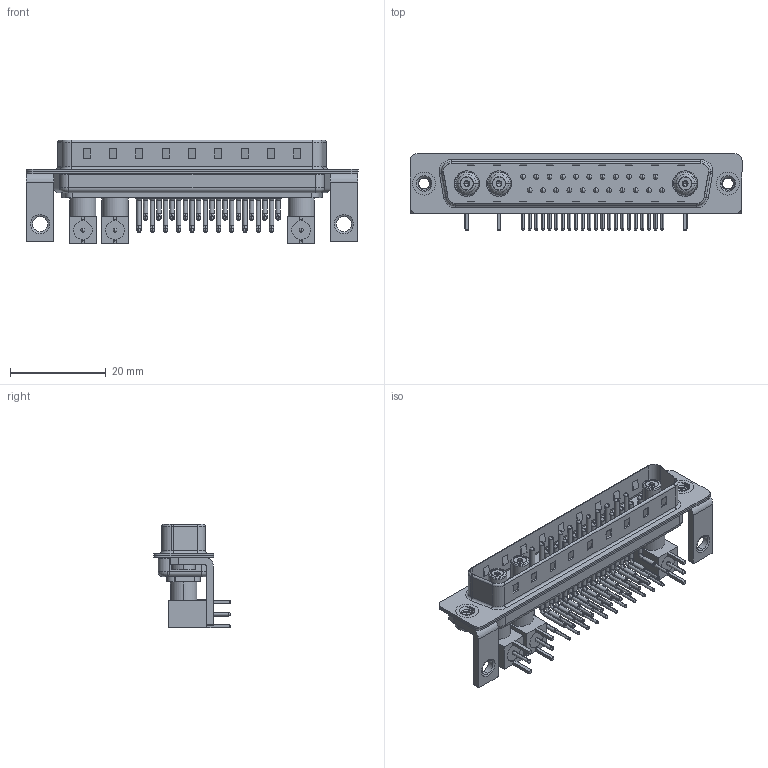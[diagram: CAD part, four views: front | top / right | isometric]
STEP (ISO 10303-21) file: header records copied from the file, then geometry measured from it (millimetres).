
FILE_DESCRIPTION (( 'STEP AP203' ), '1' );
FILE_NAME ('629-25W3640-7NC.STEP', '2022-05-16T09:23:09', ( '' ), ( '' ), 'SwSTEP 2.0', 'SolidWorks 2020', '' );
FILE_SCHEMA (( 'CONFIG_CONTROL_DESIGN' ));
Length unit declared in the file: millimetre
Products named in the file (18): 629Combo Threaded Rivet_2; Insulator RA Pin; 629Combo Shell Front_37 Contacts; Co-Ax Jack Assy_RA; 629Combo Stabilizer Bracket; 629-25W3640-7NC; 629Combo Housing_25W3; Co-Ax Jack_RA PC Tail; 629Combo Shell Rear_37 Contacts; Socket_RA; 629Combo Contact Row 2; Insulator Socket 2; RA Back Shell; Locking Collar; 629Combo Contact Row 1; Insulator Socket
Assembly tree (53 placements, depth 3):
  629-25W3640-7NC
    629Combo Housing_25W3
    629Combo Shell Rear_37 Contacts
    629Combo Shell Front_37 Contacts
    629Combo Threaded Rivet_2  x2
    629Combo Stabilizer Bracket  x2
    Co-Ax Jack Assy_RA
      Co-Ax Jack_RA PC Tail
      Insulator Socket
      Insulator Socket 2
      Locking Collar
      Socket_RA
      RA Back Shell
      Insulator RA Pin
    Co-Ax Jack Assy_RA
      Co-Ax Jack_RA PC Tail
      Insulator Socket
      Insulator Socket 2
      Locking Collar
      Socket_RA
      RA Back Shell
      Insulator RA Pin
    Co-Ax Jack Assy_RA
      Co-Ax Jack_RA PC Tail
      Insulator Socket
      Insulator Socket 2
      Locking Collar
      Socket_RA
      RA Back Shell
      Insulator RA Pin
    629Combo Contact Row 1  x11
    629Combo Contact Row 2  x11
Bounding box: 69.4 x 16 x 21.71 mm (x, y, z)
Volume: 5114.2 mm3; surface area: 13388.8 mm2
Topology: 50 solids, 50 shells, 3336 faces, 9062 edges, 5855 vertices
Faces by surface type: plane 1802, cylinder 1158, cone 161, bspline 141, torus 68, sphere 6
Entity records: 33366 total; most frequent: CARTESIAN_POINT 6813, DIRECTION 5196, ORIENTED_EDGE 4742, EDGE_CURVE 2371, AXIS2_PLACEMENT_3D 1902, VERTEX_POINT 1529, LINE 1392, VECTOR 1392
